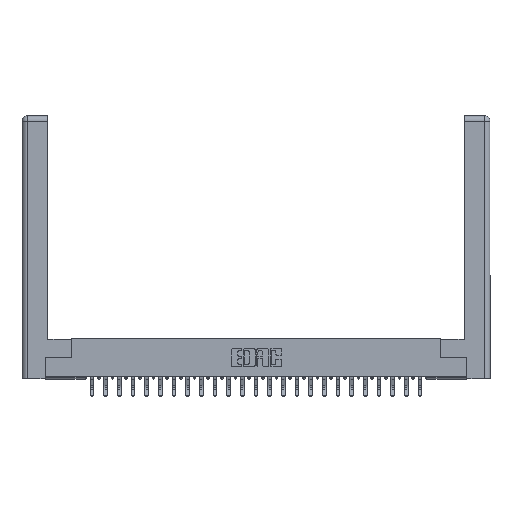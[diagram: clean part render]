
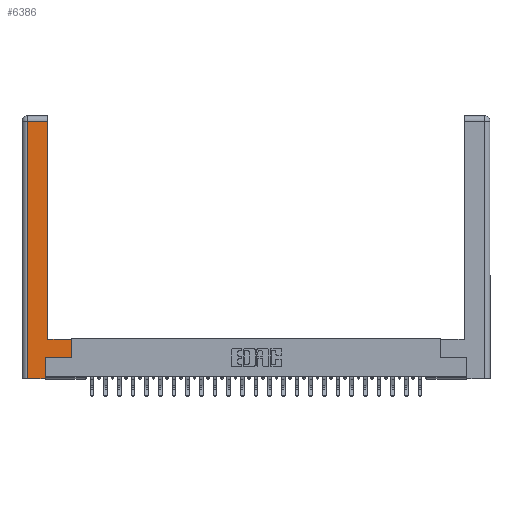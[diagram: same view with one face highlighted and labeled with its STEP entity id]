
A CAD part, top view. The second image highlights one B-rep face of the part: STEP entity #6386.
In plain terms, the highlighted planar face has unit normal (0, 0, 1).
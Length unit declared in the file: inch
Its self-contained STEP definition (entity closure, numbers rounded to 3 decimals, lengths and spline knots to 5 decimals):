
#898 = VERTEX_POINT ( 'NONE', #7922 ) ;
#2680 = VECTOR ( 'NONE', #14621, 39.37008 ) ;
#3261 = DIRECTION ( 'NONE',  ( 1., 0., 0. ) ) ;
#4317 = VERTEX_POINT ( 'NONE', #11222 ) ;
#4977 = VERTEX_POINT ( 'NONE', #28418 ) ;
#5516 = LINE ( 'NONE', #22487, #8255 ) ;
#5772 = ORIENTED_EDGE ( 'NONE', *, *, #14281, .T. ) ;
#5774 = ORIENTED_EDGE ( 'NONE', *, *, #15618, .T. ) ;
#6225 = CARTESIAN_POINT ( 'NONE',  ( 0.295, 2.94, 0. ) ) ;
#6386 = ADVANCED_FACE ( 'NONE', ( #12757 ), #26891, .F. ) ;
#7085 = DIRECTION ( 'NONE',  ( 0., 1., 0. ) ) ;
#7648 = DIRECTION ( 'NONE',  ( -1., 0., 0. ) ) ;
#7922 = CARTESIAN_POINT ( 'NONE',  ( 0.565, 0.245, 0. ) ) ;
#8255 = VECTOR ( 'NONE', #3261, 39.37008 ) ;
#8422 = DIRECTION ( 'NONE',  ( 0., 1., 0. ) ) ;
#9504 = LINE ( 'NONE', #16882, #13347 ) ;
#11222 = CARTESIAN_POINT ( 'NONE',  ( 0.0615, 2.94, 0. ) ) ;
#11855 = DIRECTION ( 'NONE',  ( -1., 0., 0. ) ) ;
#11926 = VERTEX_POINT ( 'NONE', #18784 ) ;
#12062 = DIRECTION ( 'NONE',  ( 1., 0., 0. ) ) ;
#12173 = CARTESIAN_POINT ( 'NONE',  ( 0., 0., 0. ) ) ;
#12196 = EDGE_CURVE ( 'NONE', #19683, #11926, #14367, .T. ) ;
#12464 = LINE ( 'NONE', #15375, #26664 ) ;
#12757 = FACE_OUTER_BOUND ( 'NONE', #29264, .T. ) ;
#12775 = ORIENTED_EDGE ( 'NONE', *, *, #27532, .T. ) ;
#12816 = CARTESIAN_POINT ( 'NONE',  ( 0.295, 0.45, 0. ) ) ;
#13305 = VERTEX_POINT ( 'NONE', #6225 ) ;
#13347 = VECTOR ( 'NONE', #12062, 39.37008 ) ;
#14281 = EDGE_CURVE ( 'NONE', #26354, #4977, #5516, .T. ) ;
#14367 = LINE ( 'NONE', #12816, #21255 ) ;
#14621 = DIRECTION ( 'NONE',  ( -1., 0., 0. ) ) ;
#15375 = CARTESIAN_POINT ( 'NONE',  ( 0.265, 0.245, 0. ) ) ;
#15618 = EDGE_CURVE ( 'NONE', #4317, #26354, #31348, .T. ) ;
#15702 = CARTESIAN_POINT ( 'NONE',  ( 0.565, 0.45, 0. ) ) ;
#16364 = LINE ( 'NONE', #15702, #26919 ) ;
#16882 = CARTESIAN_POINT ( 'NONE',  ( 0.565, 0.245, 0. ) ) ;
#17786 = DIRECTION ( 'NONE',  ( 0., 1., 0. ) ) ;
#17795 = ORIENTED_EDGE ( 'NONE', *, *, #24895, .T. ) ;
#18035 = ORIENTED_EDGE ( 'NONE', *, *, #22612, .T. ) ;
#18408 = DIRECTION ( 'NONE',  ( 0., -1., 0. ) ) ;
#18784 = CARTESIAN_POINT ( 'NONE',  ( 0.295, 0.45, 0. ) ) ;
#18876 = CARTESIAN_POINT ( 'NONE',  ( 0.0615, 0., 0. ) ) ;
#18988 = CARTESIAN_POINT ( 'NONE',  ( 0.0615, 0., 0. ) ) ;
#19323 = CARTESIAN_POINT ( 'NONE',  ( 0.0615, 2.94, 0. ) ) ;
#19683 = VERTEX_POINT ( 'NONE', #20562 ) ;
#20153 = EDGE_CURVE ( 'NONE', #22165, #898, #9504, .T. ) ;
#20562 = CARTESIAN_POINT ( 'NONE',  ( 0.565, 0.45, 0. ) ) ;
#20711 = VECTOR ( 'NONE', #7085, 39.37008 ) ;
#21255 = VECTOR ( 'NONE', #7648, 39.37008 ) ;
#22165 = VERTEX_POINT ( 'NONE', #27751 ) ;
#22487 = CARTESIAN_POINT ( 'NONE',  ( 0.265, 0., 0. ) ) ;
#22612 = EDGE_CURVE ( 'NONE', #11926, #13305, #30028, .T. ) ;
#23154 = VECTOR ( 'NONE', #18408, 39.37008 ) ;
#23581 = DIRECTION ( 'NONE',  ( 0., 0., -1. ) ) ;
#23970 = AXIS2_PLACEMENT_3D ( 'NONE', #12173, #23581, #11855 ) ;
#24141 = CARTESIAN_POINT ( 'NONE',  ( 0.295, 3., 0. ) ) ;
#24895 = EDGE_CURVE ( 'NONE', #898, #19683, #16364, .T. ) ;
#25361 = LINE ( 'NONE', #19323, #2680 ) ;
#26354 = VERTEX_POINT ( 'NONE', #18988 ) ;
#26664 = VECTOR ( 'NONE', #17786, 39.37008 ) ;
#26891 = PLANE ( 'NONE',  #23970 ) ;
#26919 = VECTOR ( 'NONE', #8422, 39.37008 ) ;
#27341 = ORIENTED_EDGE ( 'NONE', *, *, #12196, .T. ) ;
#27532 = EDGE_CURVE ( 'NONE', #4977, #22165, #12464, .T. ) ;
#27751 = CARTESIAN_POINT ( 'NONE',  ( 0.265, 0.245, 0. ) ) ;
#27933 = ORIENTED_EDGE ( 'NONE', *, *, #20153, .T. ) ;
#28418 = CARTESIAN_POINT ( 'NONE',  ( 0.265, 0., 0. ) ) ;
#29264 = EDGE_LOOP ( 'NONE', ( #18035, #30607, #5774, #5772, #12775, #27933, #17795, #27341 ) ) ;
#29267 = EDGE_CURVE ( 'NONE', #13305, #4317, #25361, .T. ) ;
#30028 = LINE ( 'NONE', #24141, #20711 ) ;
#30607 = ORIENTED_EDGE ( 'NONE', *, *, #29267, .T. ) ;
#31348 = LINE ( 'NONE', #18876, #23154 ) ;
